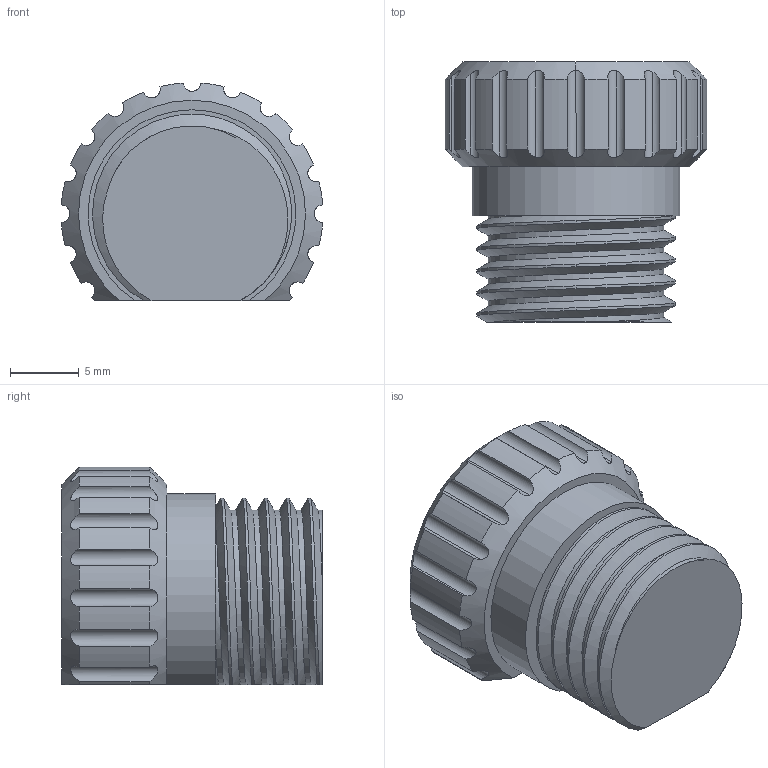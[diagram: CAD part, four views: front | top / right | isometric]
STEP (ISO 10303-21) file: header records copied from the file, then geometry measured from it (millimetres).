
FILE_DESCRIPTION (( 'STEP AP203' ), '1' );
FILE_NAME ('AF-WF-LR-PRT-008-STEP.STEP', '2020-07-21T18:16:19', ( '' ), ( '' ), 'SwSTEP 2.0', 'SolidWorks 2018', '' );
FILE_SCHEMA (( 'CONFIG_CONTROL_DESIGN' ));
Length unit declared in the file: inch
Products named in the file (1): AF-WF-LR-PRT-008-STEP
Bounding box: 19.01 x 18.92 x 15.85 mm (x, y, z)
Volume: 3508.9 mm3; surface area: 1648.1 mm2
Topology: 1 solids, 1 shells, 84 faces, 242 edges, 161 vertices
Faces by surface type: cylinder 55, bspline 18, plane 8, cone 3
Entity records: 7468 total; most frequent: CARTESIAN_POINT 5495, ORIENTED_EDGE 484, DIRECTION 298, EDGE_CURVE 242, VERTEX_POINT 161, AXIS2_PLACEMENT_3D 112, EDGE_LOOP 85, ADVANCED_FACE 84
